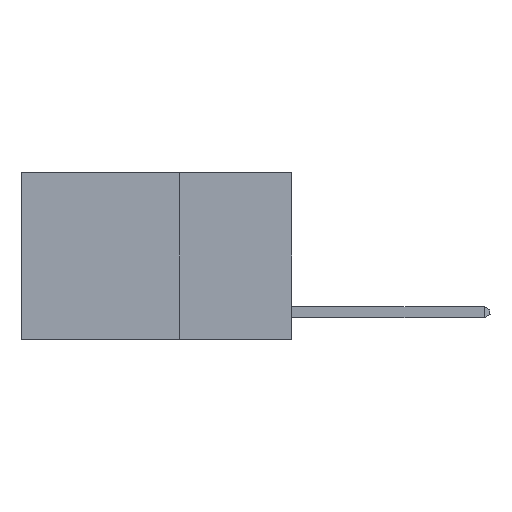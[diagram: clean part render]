
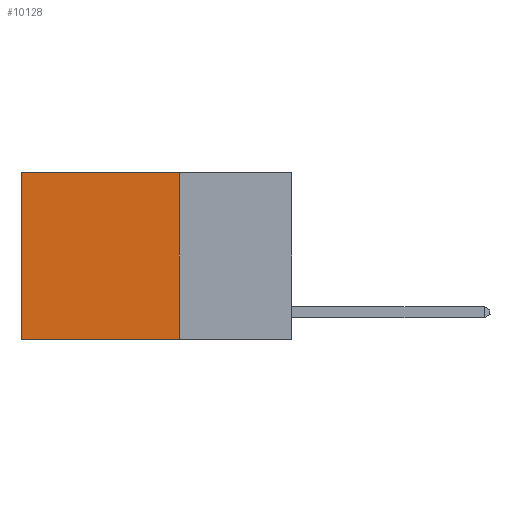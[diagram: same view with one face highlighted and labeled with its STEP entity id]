
A CAD part, left-side view. The second image highlights one B-rep face of the part: STEP entity #10128.
In plain terms, the highlighted planar face has unit normal (-1, 0, 0).
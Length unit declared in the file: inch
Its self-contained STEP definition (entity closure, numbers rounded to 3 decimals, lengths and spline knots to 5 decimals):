
#75 = EDGE_CURVE ( 'NONE', #13401, #3800, #9898, .T. ) ;
#529 = CARTESIAN_POINT ( 'NONE',  ( 0.2625, 0.6, 0. ) ) ;
#690 = VECTOR ( 'NONE', #6073, 39.37008 ) ;
#1433 = AXIS2_PLACEMENT_3D ( 'NONE', #7698, #8791, #2197 ) ;
#2197 = DIRECTION ( 'NONE',  ( 0., 0., -1. ) ) ;
#2553 = EDGE_CURVE ( 'NONE', #10540, #9235, #7512, .T. ) ;
#2672 = LINE ( 'NONE', #9899, #8196 ) ;
#3214 = CARTESIAN_POINT ( 'NONE',  ( 0.2625, 0.6, 0. ) ) ;
#3395 = EDGE_CURVE ( 'NONE', #10540, #13401, #2672, .T. ) ;
#3800 = VERTEX_POINT ( 'NONE', #10082 ) ;
#3976 = DIRECTION ( 'NONE',  ( 0., 1., 0. ) ) ;
#4939 = EDGE_CURVE ( 'NONE', #9235, #3800, #6626, .T. ) ;
#5064 = ORIENTED_EDGE ( 'NONE', *, *, #4939, .T. ) ;
#6073 = DIRECTION ( 'NONE',  ( 0., 0., -1. ) ) ;
#6626 = LINE ( 'NONE', #529, #690 ) ;
#6949 = VECTOR ( 'NONE', #3976, 39.37008 ) ;
#7512 = LINE ( 'NONE', #9082, #10144 ) ;
#7532 = CARTESIAN_POINT ( 'NONE',  ( 0.2625, 0.25, 0. ) ) ;
#7698 = CARTESIAN_POINT ( 'NONE',  ( 0.2625, 0.25, 0. ) ) ;
#8196 = VECTOR ( 'NONE', #9759, 39.37008 ) ;
#8791 = DIRECTION ( 'NONE',  ( 1., 0., 0. ) ) ;
#8952 = DIRECTION ( 'NONE',  ( 0., 1., 0. ) ) ;
#9082 = CARTESIAN_POINT ( 'NONE',  ( 0.2625, 0.25, 0. ) ) ;
#9235 = VERTEX_POINT ( 'NONE', #3214 ) ;
#9759 = DIRECTION ( 'NONE',  ( 0., 0., -1. ) ) ;
#9898 = LINE ( 'NONE', #12452, #6949 ) ;
#9899 = CARTESIAN_POINT ( 'NONE',  ( 0.2625, 0.25, 0. ) ) ;
#10075 = ORIENTED_EDGE ( 'NONE', *, *, #2553, .T. ) ;
#10082 = CARTESIAN_POINT ( 'NONE',  ( 0.2625, 0.6, -0.37 ) ) ;
#10128 = ADVANCED_FACE ( 'NONE', ( #14377 ), #14418, .F. ) ;
#10144 = VECTOR ( 'NONE', #8952, 39.37008 ) ;
#10540 = VERTEX_POINT ( 'NONE', #7532 ) ;
#10591 = EDGE_LOOP ( 'NONE', ( #5064, #14402, #12766, #10075 ) ) ;
#12452 = CARTESIAN_POINT ( 'NONE',  ( 0.2625, 0.25, -0.37 ) ) ;
#12766 = ORIENTED_EDGE ( 'NONE', *, *, #3395, .F. ) ;
#13401 = VERTEX_POINT ( 'NONE', #14425 ) ;
#14377 = FACE_OUTER_BOUND ( 'NONE', #10591, .T. ) ;
#14402 = ORIENTED_EDGE ( 'NONE', *, *, #75, .F. ) ;
#14418 = PLANE ( 'NONE',  #1433 ) ;
#14425 = CARTESIAN_POINT ( 'NONE',  ( 0.2625, 0.25, -0.37 ) ) ;
